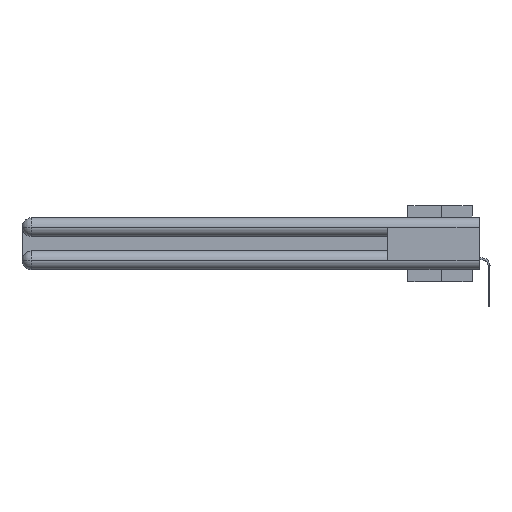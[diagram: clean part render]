
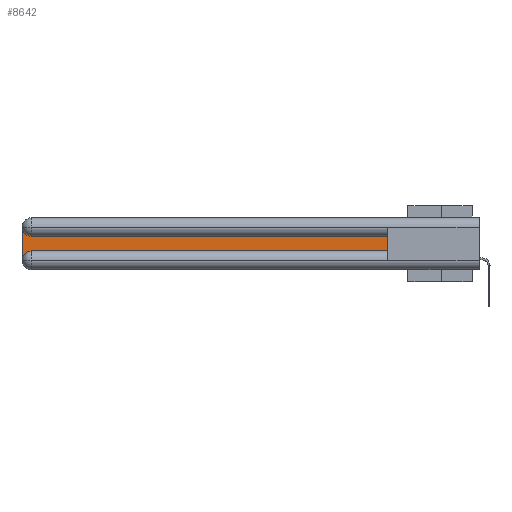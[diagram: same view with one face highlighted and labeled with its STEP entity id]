
A CAD part, left-side view. The second image highlights one B-rep face of the part: STEP entity #8642.
In plain terms, the highlighted planar face has unit normal (-1, 0, 0).
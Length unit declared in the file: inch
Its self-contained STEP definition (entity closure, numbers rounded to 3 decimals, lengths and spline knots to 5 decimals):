
#377 = EDGE_LOOP ( 'NONE', ( #24279, #33703, #25150, #14889, #36497, #26001 ) ) ;
#842 = VERTEX_POINT ( 'NONE', #6479 ) ;
#2814 = PLANE ( 'NONE',  #35398 ) ;
#3502 = CARTESIAN_POINT ( 'NONE',  ( 0.075, 0.6, -0.2175 ) ) ;
#4073 = EDGE_CURVE ( 'NONE', #38691, #17178, #28455, .T. ) ;
#5428 = EDGE_CURVE ( 'NONE', #5847, #6863, #36763, .T. ) ;
#5598 = VECTOR ( 'NONE', #17060, 39.37008 ) ;
#5847 = VERTEX_POINT ( 'NONE', #11183 ) ;
#6150 = AXIS2_PLACEMENT_3D ( 'NONE', #37713, #28519, #19739 ) ;
#6377 = DIRECTION ( 'NONE',  ( 0., 0., -1. ) ) ;
#6479 = CARTESIAN_POINT ( 'NONE',  ( 0.075, 3., -0.0625 ) ) ;
#6753 = CARTESIAN_POINT ( 'NONE',  ( 0.075, 2.94, -0.0625 ) ) ;
#6863 = VERTEX_POINT ( 'NONE', #29272 ) ;
#8040 = DIRECTION ( 'NONE',  ( 0., 0., -1. ) ) ;
#8252 = CARTESIAN_POINT ( 'NONE',  ( 0.075, 3., -0.1225 ) ) ;
#8642 = ADVANCED_FACE ( 'NONE', ( #32803 ), #2814, .F. ) ;
#11183 = CARTESIAN_POINT ( 'NONE',  ( 0.075, 3., -0.2775 ) ) ;
#14256 = CARTESIAN_POINT ( 'NONE',  ( 0.075, 0.6, -0.1225 ) ) ;
#14889 = ORIENTED_EDGE ( 'NONE', *, *, #5428, .T. ) ;
#15724 = DIRECTION ( 'NONE',  ( 0., -1., 0. ) ) ;
#15871 = EDGE_CURVE ( 'NONE', #17178, #28544, #32613, .T. ) ;
#17060 = DIRECTION ( 'NONE',  ( 0., 1., 0. ) ) ;
#17178 = VERTEX_POINT ( 'NONE', #14256 ) ;
#17447 = CARTESIAN_POINT ( 'NONE',  ( 0.075, 0.6, -0.1225 ) ) ;
#19692 = VECTOR ( 'NONE', #32836, 39.37008 ) ;
#19739 = DIRECTION ( 'NONE',  ( 0., 0., -1. ) ) ;
#20170 = AXIS2_PLACEMENT_3D ( 'NONE', #6753, #31137, #6377 ) ;
#21346 = CARTESIAN_POINT ( 'NONE',  ( 0.075, 0.6, -0.2175 ) ) ;
#21679 = CARTESIAN_POINT ( 'NONE',  ( 0.075, 0.6, -0.2175 ) ) ;
#22058 = LINE ( 'NONE', #29266, #19692 ) ;
#22709 = EDGE_CURVE ( 'NONE', #6863, #38691, #25698, .T. ) ;
#24279 = ORIENTED_EDGE ( 'NONE', *, *, #15871, .T. ) ;
#25150 = ORIENTED_EDGE ( 'NONE', *, *, #25690, .T. ) ;
#25690 = EDGE_CURVE ( 'NONE', #842, #5847, #22058, .T. ) ;
#25698 = LINE ( 'NONE', #3502, #35671 ) ;
#26001 = ORIENTED_EDGE ( 'NONE', *, *, #4073, .T. ) ;
#26991 = VECTOR ( 'NONE', #37239, 39.37008 ) ;
#27001 = DIRECTION ( 'NONE',  ( 1., 0., 0. ) ) ;
#28455 = LINE ( 'NONE', #21679, #26991 ) ;
#28519 = DIRECTION ( 'NONE',  ( 1., 0., 0. ) ) ;
#28544 = VERTEX_POINT ( 'NONE', #32090 ) ;
#29266 = CARTESIAN_POINT ( 'NONE',  ( 0.075, 3., -0.2175 ) ) ;
#29272 = CARTESIAN_POINT ( 'NONE',  ( 0.075, 2.94, -0.2175 ) ) ;
#31137 = DIRECTION ( 'NONE',  ( 1., 0., 0. ) ) ;
#32090 = CARTESIAN_POINT ( 'NONE',  ( 0.075, 2.94, -0.1225 ) ) ;
#32613 = LINE ( 'NONE', #17447, #5598 ) ;
#32803 = FACE_OUTER_BOUND ( 'NONE', #377, .T. ) ;
#32836 = DIRECTION ( 'NONE',  ( 0., 0., -1. ) ) ;
#33703 = ORIENTED_EDGE ( 'NONE', *, *, #35775, .T. ) ;
#35398 = AXIS2_PLACEMENT_3D ( 'NONE', #8252, #27001, #8040 ) ;
#35671 = VECTOR ( 'NONE', #15724, 39.37008 ) ;
#35775 = EDGE_CURVE ( 'NONE', #28544, #842, #36756, .T. ) ;
#36497 = ORIENTED_EDGE ( 'NONE', *, *, #22709, .T. ) ;
#36756 = CIRCLE ( 'NONE', #20170, 0.06 ) ;
#36763 = CIRCLE ( 'NONE', #6150, 0.06 ) ;
#37239 = DIRECTION ( 'NONE',  ( 0., 0., 1. ) ) ;
#37713 = CARTESIAN_POINT ( 'NONE',  ( 0.075, 2.94, -0.2775 ) ) ;
#38691 = VERTEX_POINT ( 'NONE', #21346 ) ;
